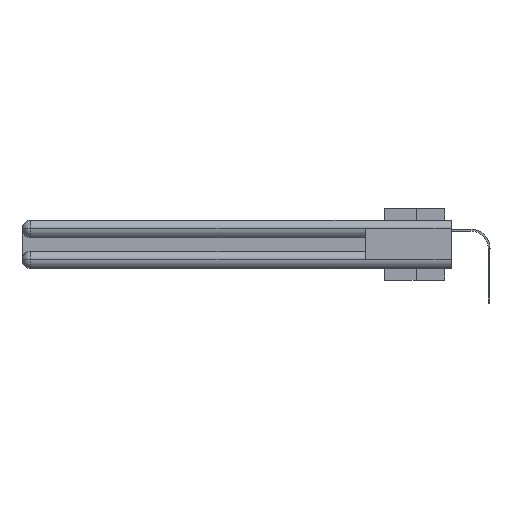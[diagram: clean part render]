
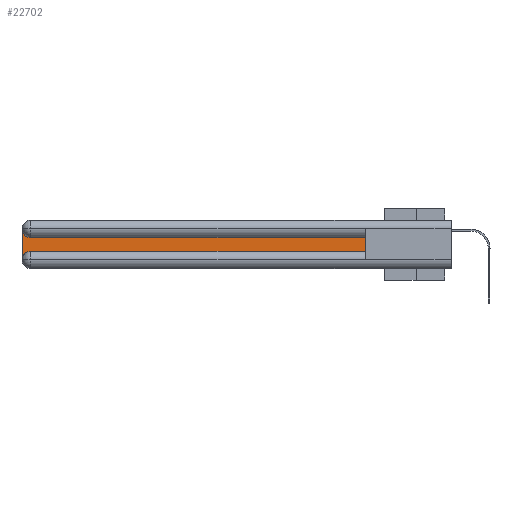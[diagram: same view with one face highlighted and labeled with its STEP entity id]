
A CAD part, left-side view. The second image highlights one B-rep face of the part: STEP entity #22702.
In plain terms, the highlighted planar face has unit normal (-1, 0, 0).
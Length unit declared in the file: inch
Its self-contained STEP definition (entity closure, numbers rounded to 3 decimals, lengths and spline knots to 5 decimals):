
#164 = VERTEX_POINT ( 'NONE', #3768 ) ;
#606 = EDGE_CURVE ( 'NONE', #22706, #23788, #17899, .T. ) ;
#1038 = VECTOR ( 'NONE', #19033, 39.37008 ) ;
#1349 = DIRECTION ( 'NONE',  ( 0., 1., 0. ) ) ;
#2016 = LINE ( 'NONE', #31089, #1038 ) ;
#2036 = EDGE_CURVE ( 'NONE', #164, #13581, #2290, .T. ) ;
#2290 = LINE ( 'NONE', #19327, #20533 ) ;
#3171 = DIRECTION ( 'NONE',  ( 0., -1., 0. ) ) ;
#3258 = DIRECTION ( 'NONE',  ( 1., 0., 0. ) ) ;
#3359 = ORIENTED_EDGE ( 'NONE', *, *, #9162, .T. ) ;
#3768 = CARTESIAN_POINT ( 'NONE',  ( 0.075, 3., -0.0625 ) ) ;
#5754 = ORIENTED_EDGE ( 'NONE', *, *, #20068, .T. ) ;
#5821 = CARTESIAN_POINT ( 'NONE',  ( 0.075, 0.6, -0.1225 ) ) ;
#6343 = AXIS2_PLACEMENT_3D ( 'NONE', #14569, #26936, #24238 ) ;
#7564 = EDGE_CURVE ( 'NONE', #13581, #28526, #18593, .T. ) ;
#9162 = EDGE_CURVE ( 'NONE', #28526, #17053, #17660, .T. ) ;
#10740 = CARTESIAN_POINT ( 'NONE',  ( 0.075, 2.94, -0.1225 ) ) ;
#11049 = CARTESIAN_POINT ( 'NONE',  ( 0.075, 2.94, -0.2175 ) ) ;
#13127 = PLANE ( 'NONE',  #22424 ) ;
#13581 = VERTEX_POINT ( 'NONE', #13940 ) ;
#13658 = EDGE_CURVE ( 'NONE', #23788, #164, #13934, .T. ) ;
#13894 = CARTESIAN_POINT ( 'NONE',  ( 0.075, 0.6, -0.2175 ) ) ;
#13934 = CIRCLE ( 'NONE', #6343, 0.06 ) ;
#13940 = CARTESIAN_POINT ( 'NONE',  ( 0.075, 3., -0.2775 ) ) ;
#14569 = CARTESIAN_POINT ( 'NONE',  ( 0.075, 2.94, -0.0625 ) ) ;
#15356 = FACE_OUTER_BOUND ( 'NONE', #15415, .T. ) ;
#15415 = EDGE_LOOP ( 'NONE', ( #16136, #19566, #25906, #21470, #3359, #5754 ) ) ;
#16107 = DIRECTION ( 'NONE',  ( 1., 0., 0. ) ) ;
#16136 = ORIENTED_EDGE ( 'NONE', *, *, #606, .T. ) ;
#17053 = VERTEX_POINT ( 'NONE', #13894 ) ;
#17660 = LINE ( 'NONE', #26869, #25240 ) ;
#17899 = LINE ( 'NONE', #5821, #20408 ) ;
#18386 = DIRECTION ( 'NONE',  ( 0., 0., -1. ) ) ;
#18593 = CIRCLE ( 'NONE', #30758, 0.06 ) ;
#19033 = DIRECTION ( 'NONE',  ( 0., 0., 1. ) ) ;
#19327 = CARTESIAN_POINT ( 'NONE',  ( 0.075, 3., -0.2175 ) ) ;
#19566 = ORIENTED_EDGE ( 'NONE', *, *, #13658, .T. ) ;
#20068 = EDGE_CURVE ( 'NONE', #17053, #22706, #2016, .T. ) ;
#20408 = VECTOR ( 'NONE', #1349, 39.37008 ) ;
#20533 = VECTOR ( 'NONE', #31068, 39.37008 ) ;
#21470 = ORIENTED_EDGE ( 'NONE', *, *, #7564, .T. ) ;
#22424 = AXIS2_PLACEMENT_3D ( 'NONE', #25022, #3258, #18386 ) ;
#22702 = ADVANCED_FACE ( 'NONE', ( #15356 ), #13127, .F. ) ;
#22706 = VERTEX_POINT ( 'NONE', #28386 ) ;
#23788 = VERTEX_POINT ( 'NONE', #10740 ) ;
#24238 = DIRECTION ( 'NONE',  ( 0., 0., -1. ) ) ;
#25022 = CARTESIAN_POINT ( 'NONE',  ( 0.075, 3., -0.1225 ) ) ;
#25240 = VECTOR ( 'NONE', #3171, 39.37008 ) ;
#25771 = DIRECTION ( 'NONE',  ( 0., 0., -1. ) ) ;
#25906 = ORIENTED_EDGE ( 'NONE', *, *, #2036, .T. ) ;
#26869 = CARTESIAN_POINT ( 'NONE',  ( 0.075, 0.6, -0.2175 ) ) ;
#26936 = DIRECTION ( 'NONE',  ( 1., 0., 0. ) ) ;
#28165 = CARTESIAN_POINT ( 'NONE',  ( 0.075, 2.94, -0.2775 ) ) ;
#28386 = CARTESIAN_POINT ( 'NONE',  ( 0.075, 0.6, -0.1225 ) ) ;
#28526 = VERTEX_POINT ( 'NONE', #11049 ) ;
#30758 = AXIS2_PLACEMENT_3D ( 'NONE', #28165, #16107, #25771 ) ;
#31068 = DIRECTION ( 'NONE',  ( 0., 0., -1. ) ) ;
#31089 = CARTESIAN_POINT ( 'NONE',  ( 0.075, 0.6, -0.2175 ) ) ;
